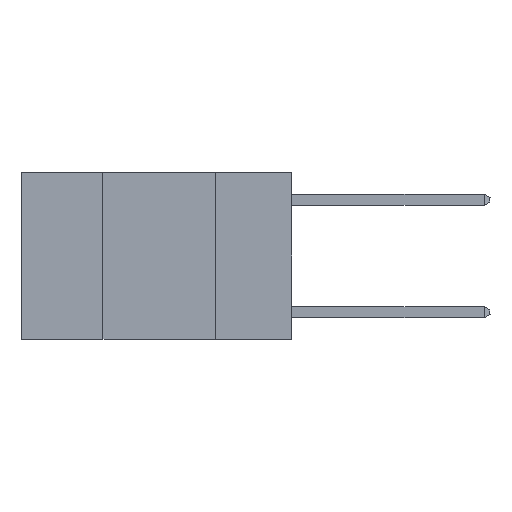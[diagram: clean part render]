
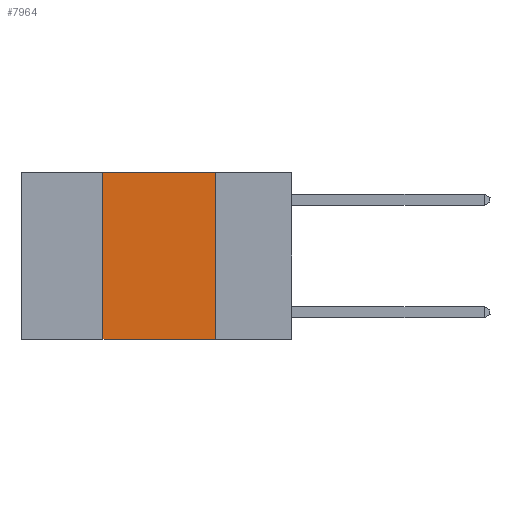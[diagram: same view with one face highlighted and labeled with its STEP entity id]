
A CAD part, left-side view. The second image highlights one B-rep face of the part: STEP entity #7964.
In plain terms, the highlighted planar face has unit normal (-1, 0, 0).
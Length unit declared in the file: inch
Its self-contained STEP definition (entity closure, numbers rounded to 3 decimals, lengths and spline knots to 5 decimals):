
#391 = CARTESIAN_POINT ( 'NONE',  ( 0., 0.17, 0. ) ) ;
#610 = PLANE ( 'NONE',  #9796 ) ;
#1258 = EDGE_CURVE ( 'NONE', #6356, #9047, #15238, .T. ) ;
#2901 = CARTESIAN_POINT ( 'NONE',  ( 0., 0.17, -0.37 ) ) ;
#3412 = DIRECTION ( 'NONE',  ( 0., -1., 0. ) ) ;
#3568 = VERTEX_POINT ( 'NONE', #10889 ) ;
#3723 = DIRECTION ( 'NONE',  ( 0., 0., -1. ) ) ;
#4698 = DIRECTION ( 'NONE',  ( 0., -1., 0. ) ) ;
#5016 = LINE ( 'NONE', #11454, #11916 ) ;
#5562 = EDGE_LOOP ( 'NONE', ( #7741, #17311, #15590, #15094 ) ) ;
#5711 = CARTESIAN_POINT ( 'NONE',  ( 0., 0.42, 0. ) ) ;
#5885 = EDGE_CURVE ( 'NONE', #3568, #12459, #15708, .T. ) ;
#5892 = CARTESIAN_POINT ( 'NONE',  ( 0., 0.17, 0. ) ) ;
#6356 = VERTEX_POINT ( 'NONE', #5892 ) ;
#6964 = CARTESIAN_POINT ( 'NONE',  ( 0., 0.6, -0.37 ) ) ;
#7176 = CARTESIAN_POINT ( 'NONE',  ( 0., 0.6, 0. ) ) ;
#7250 = VECTOR ( 'NONE', #7335, 39.37008 ) ;
#7335 = DIRECTION ( 'NONE',  ( 0., 0., 1. ) ) ;
#7741 = ORIENTED_EDGE ( 'NONE', *, *, #1258, .F. ) ;
#7870 = EDGE_CURVE ( 'NONE', #3568, #9047, #15244, .T. ) ;
#7964 = ADVANCED_FACE ( 'NONE', ( #12008 ), #610, .F. ) ;
#9047 = VERTEX_POINT ( 'NONE', #2901 ) ;
#9796 = AXIS2_PLACEMENT_3D ( 'NONE', #7176, #18617, #20109 ) ;
#10521 = EDGE_CURVE ( 'NONE', #12459, #6356, #5016, .T. ) ;
#10889 = CARTESIAN_POINT ( 'NONE',  ( 0., 0.42, -0.37 ) ) ;
#11454 = CARTESIAN_POINT ( 'NONE',  ( 0., 0.6, 0. ) ) ;
#11916 = VECTOR ( 'NONE', #4698, 39.37008 ) ;
#12008 = FACE_OUTER_BOUND ( 'NONE', #5562, .T. ) ;
#12459 = VERTEX_POINT ( 'NONE', #19964 ) ;
#15094 = ORIENTED_EDGE ( 'NONE', *, *, #7870, .T. ) ;
#15238 = LINE ( 'NONE', #391, #17623 ) ;
#15244 = LINE ( 'NONE', #6964, #18817 ) ;
#15590 = ORIENTED_EDGE ( 'NONE', *, *, #5885, .F. ) ;
#15708 = LINE ( 'NONE', #5711, #7250 ) ;
#17311 = ORIENTED_EDGE ( 'NONE', *, *, #10521, .F. ) ;
#17623 = VECTOR ( 'NONE', #3723, 39.37008 ) ;
#18617 = DIRECTION ( 'NONE',  ( 1., 0., 0. ) ) ;
#18817 = VECTOR ( 'NONE', #3412, 39.37008 ) ;
#19964 = CARTESIAN_POINT ( 'NONE',  ( 0., 0.42, 0. ) ) ;
#20109 = DIRECTION ( 'NONE',  ( 0., 0., -1. ) ) ;
